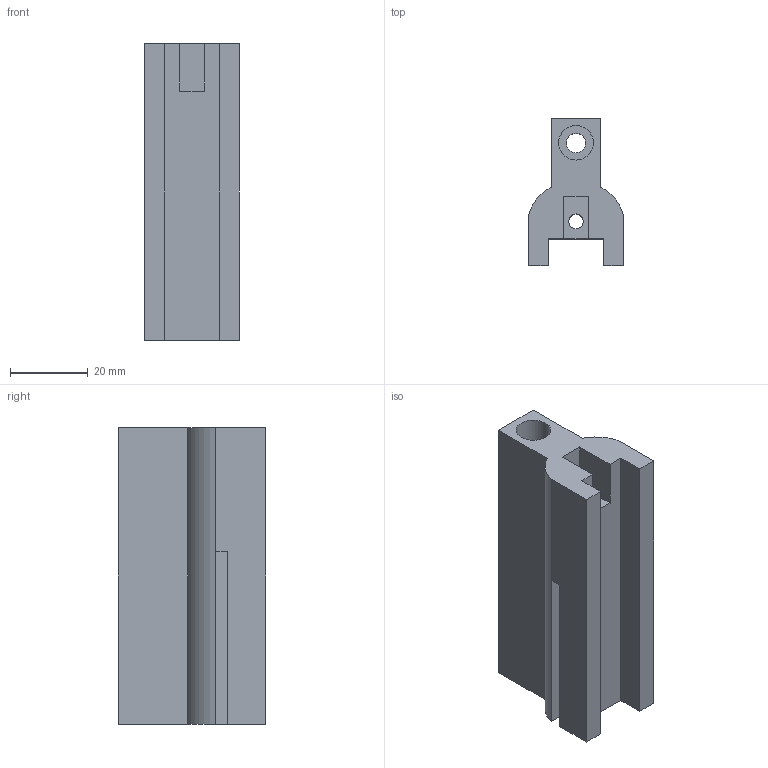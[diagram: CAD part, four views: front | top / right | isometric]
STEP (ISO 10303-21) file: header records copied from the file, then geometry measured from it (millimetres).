
FILE_DESCRIPTION((''),'2;1');
FILE_NAME('BOLT','2013-06-13T',('fireraisr'),(''),'PRO/ENGINEER BY PARAMETRIC TECHNOLOGY CORPORATION, 2007450','PRO/ENGINEER BY PARAMETRIC TECHNOLOGY CORPORATION, 2007450','');
FILE_SCHEMA(('CONFIG_CONTROL_DESIGN'));
Length unit declared in the file: inch
Products named in the file (1): BOLT
Bounding box: 24.38 x 37.85 x 76.2 mm (x, y, z)
Volume: 39306.9 mm3; surface area: 14499.3 mm2
Topology: 1 solids, 1 shells, 32 faces, 84 edges, 56 vertices
Faces by surface type: plane 22, cylinder 8, extrusion 2
Entity records: 1046 total; most frequent: CARTESIAN_POINT 188, ORIENTED_EDGE 168, DIRECTION 162, EDGE_CURVE 84, VECTOR 66, LINE 64, VERTEX_POINT 56, AXIS2_PLACEMENT_3D 48
